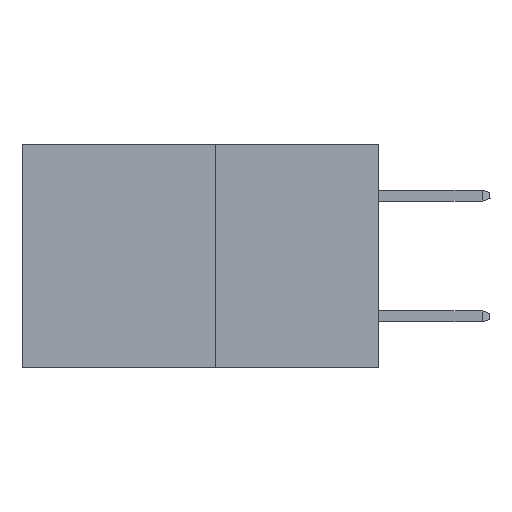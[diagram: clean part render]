
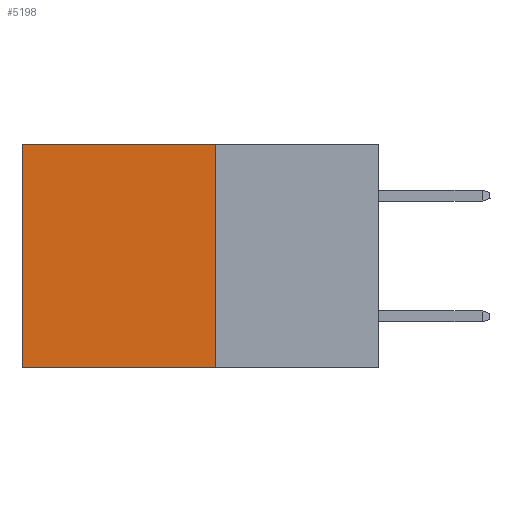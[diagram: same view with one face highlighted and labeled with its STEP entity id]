
A CAD part, left-side view. The second image highlights one B-rep face of the part: STEP entity #5198.
In plain terms, the highlighted planar face has unit normal (-1, 0, 0).
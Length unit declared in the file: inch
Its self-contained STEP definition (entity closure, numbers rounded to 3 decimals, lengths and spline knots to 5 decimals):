
#1192 = VECTOR ( 'NONE', #11224, 39.37008 ) ;
#1322 = VECTOR ( 'NONE', #13988, 39.37008 ) ;
#1567 = EDGE_CURVE ( 'NONE', #14018, #1600, #1611, .T. ) ;
#1600 = VERTEX_POINT ( 'NONE', #8334 ) ;
#1611 = LINE ( 'NONE', #10880, #1192 ) ;
#1878 = CARTESIAN_POINT ( 'NONE',  ( 0.277, 0.27, -0.37 ) ) ;
#1909 = VECTOR ( 'NONE', #3277, 39.37008 ) ;
#2825 = AXIS2_PLACEMENT_3D ( 'NONE', #8619, #8568, #8523 ) ;
#2955 = EDGE_LOOP ( 'NONE', ( #3397, #3453, #3536, #3667 ) ) ;
#3277 = DIRECTION ( 'NONE',  ( 0., 1., 0. ) ) ;
#3293 = CARTESIAN_POINT ( 'NONE',  ( 0.277, 0.27, -0.37 ) ) ;
#3397 = ORIENTED_EDGE ( 'NONE', *, *, #3830, .T. ) ;
#3416 = FACE_OUTER_BOUND ( 'NONE', #2955, .T. ) ;
#3453 = ORIENTED_EDGE ( 'NONE', *, *, #7957, .F. ) ;
#3536 = ORIENTED_EDGE ( 'NONE', *, *, #5080, .F. ) ;
#3667 = ORIENTED_EDGE ( 'NONE', *, *, #1567, .T. ) ;
#3830 = EDGE_CURVE ( 'NONE', #1600, #10654, #12835, .T. ) ;
#5049 = CARTESIAN_POINT ( 'NONE',  ( 0.277, 0.59, -0.37 ) ) ;
#5080 = EDGE_CURVE ( 'NONE', #14018, #13183, #10870, .T. ) ;
#5198 = ADVANCED_FACE ( 'NONE', ( #3416 ), #8633, .F. ) ;
#5511 = CARTESIAN_POINT ( 'NONE',  ( 0.277, 0.59, -0.37 ) ) ;
#7957 = EDGE_CURVE ( 'NONE', #13183, #10654, #10907, .T. ) ;
#8334 = CARTESIAN_POINT ( 'NONE',  ( 0.277, 0.59, 0. ) ) ;
#8523 = DIRECTION ( 'NONE',  ( 0., 0., -1. ) ) ;
#8568 = DIRECTION ( 'NONE',  ( 1., 0., 0. ) ) ;
#8619 = CARTESIAN_POINT ( 'NONE',  ( 0.277, 0.27, -0.37 ) ) ;
#8633 = PLANE ( 'NONE',  #2825 ) ;
#10126 = DIRECTION ( 'NONE',  ( 0., 0., -1. ) ) ;
#10188 = CARTESIAN_POINT ( 'NONE',  ( 0.277, 0.27, -0.37 ) ) ;
#10654 = VERTEX_POINT ( 'NONE', #5049 ) ;
#10779 = CARTESIAN_POINT ( 'NONE',  ( 0.277, 0.27, 0. ) ) ;
#10870 = LINE ( 'NONE', #10188, #12963 ) ;
#10880 = CARTESIAN_POINT ( 'NONE',  ( 0.277, 0.27, 0. ) ) ;
#10907 = LINE ( 'NONE', #3293, #1909 ) ;
#11224 = DIRECTION ( 'NONE',  ( 0., 1., 0. ) ) ;
#12835 = LINE ( 'NONE', #5511, #1322 ) ;
#12963 = VECTOR ( 'NONE', #10126, 39.37008 ) ;
#13183 = VERTEX_POINT ( 'NONE', #1878 ) ;
#13988 = DIRECTION ( 'NONE',  ( 0., 0., -1. ) ) ;
#14018 = VERTEX_POINT ( 'NONE', #10779 ) ;
